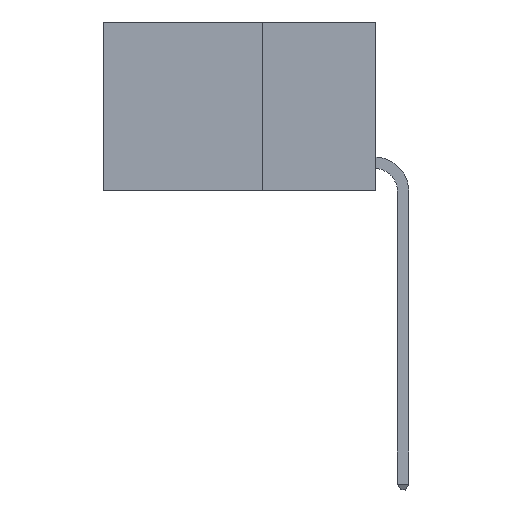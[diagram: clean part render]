
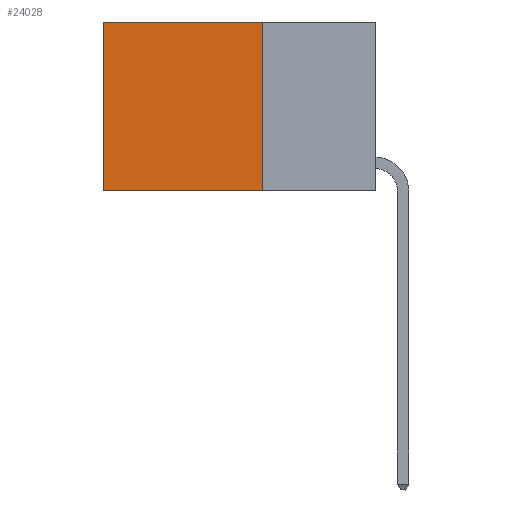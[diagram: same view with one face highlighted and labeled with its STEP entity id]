
A CAD part, left-side view. The second image highlights one B-rep face of the part: STEP entity #24028.
In plain terms, the highlighted planar face has unit normal (-1, 0, 0).
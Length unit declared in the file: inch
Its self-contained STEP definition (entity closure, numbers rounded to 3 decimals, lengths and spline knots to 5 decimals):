
#1612 = CARTESIAN_POINT ( 'NONE',  ( 0.2625, 0.25, 0. ) ) ;
#2170 = ORIENTED_EDGE ( 'NONE', *, *, #19292, .T. ) ;
#2594 = VERTEX_POINT ( 'NONE', #27050 ) ;
#2614 = VECTOR ( 'NONE', #13626, 39.37008 ) ;
#5515 = VERTEX_POINT ( 'NONE', #5844 ) ;
#5844 = CARTESIAN_POINT ( 'NONE',  ( 0.2625, 0.6, 0. ) ) ;
#6332 = ORIENTED_EDGE ( 'NONE', *, *, #13700, .F. ) ;
#7357 = DIRECTION ( 'NONE',  ( 0., 0., -1. ) ) ;
#7783 = CARTESIAN_POINT ( 'NONE',  ( 0.2625, 0.25, -0.37 ) ) ;
#7795 = LINE ( 'NONE', #9326, #2614 ) ;
#7970 = DIRECTION ( 'NONE',  ( 1., 0., 0. ) ) ;
#9326 = CARTESIAN_POINT ( 'NONE',  ( 0.2625, 0.6, 0. ) ) ;
#9341 = EDGE_CURVE ( 'NONE', #5515, #2594, #7795, .T. ) ;
#11223 = EDGE_CURVE ( 'NONE', #26230, #23966, #27619, .T. ) ;
#11469 = VECTOR ( 'NONE', #7357, 39.37008 ) ;
#11917 = DIRECTION ( 'NONE',  ( 0., 1., 0. ) ) ;
#12187 = LINE ( 'NONE', #22518, #21495 ) ;
#13134 = LINE ( 'NONE', #25694, #18106 ) ;
#13626 = DIRECTION ( 'NONE',  ( 0., 0., -1. ) ) ;
#13700 = EDGE_CURVE ( 'NONE', #23966, #2594, #12187, .T. ) ;
#15348 = ORIENTED_EDGE ( 'NONE', *, *, #11223, .F. ) ;
#16561 = CARTESIAN_POINT ( 'NONE',  ( 0.2625, 0.25, 0. ) ) ;
#17020 = EDGE_LOOP ( 'NONE', ( #19881, #6332, #15348, #2170 ) ) ;
#17525 = FACE_OUTER_BOUND ( 'NONE', #17020, .T. ) ;
#18106 = VECTOR ( 'NONE', #27727, 39.37008 ) ;
#18708 = PLANE ( 'NONE',  #22709 ) ;
#19292 = EDGE_CURVE ( 'NONE', #26230, #5515, #13134, .T. ) ;
#19881 = ORIENTED_EDGE ( 'NONE', *, *, #9341, .T. ) ;
#21495 = VECTOR ( 'NONE', #11917, 39.37008 ) ;
#22402 = CARTESIAN_POINT ( 'NONE',  ( 0.2625, 0.25, 0. ) ) ;
#22518 = CARTESIAN_POINT ( 'NONE',  ( 0.2625, 0.25, -0.37 ) ) ;
#22709 = AXIS2_PLACEMENT_3D ( 'NONE', #16561, #7970, #22977 ) ;
#22977 = DIRECTION ( 'NONE',  ( 0., 0., -1. ) ) ;
#23966 = VERTEX_POINT ( 'NONE', #7783 ) ;
#24028 = ADVANCED_FACE ( 'NONE', ( #17525 ), #18708, .F. ) ;
#25694 = CARTESIAN_POINT ( 'NONE',  ( 0.2625, 0.25, 0. ) ) ;
#26230 = VERTEX_POINT ( 'NONE', #1612 ) ;
#27050 = CARTESIAN_POINT ( 'NONE',  ( 0.2625, 0.6, -0.37 ) ) ;
#27619 = LINE ( 'NONE', #22402, #11469 ) ;
#27727 = DIRECTION ( 'NONE',  ( 0., 1., 0. ) ) ;
